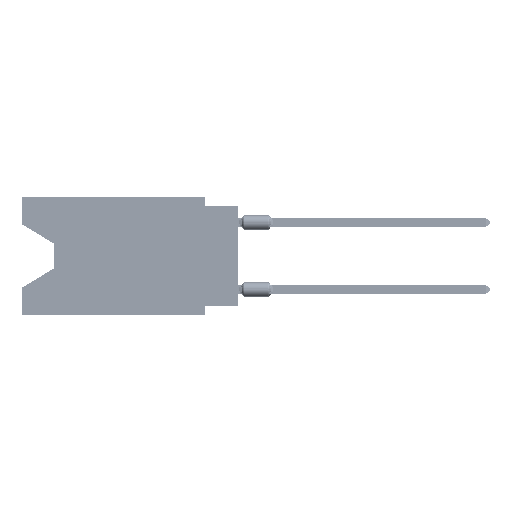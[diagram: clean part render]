
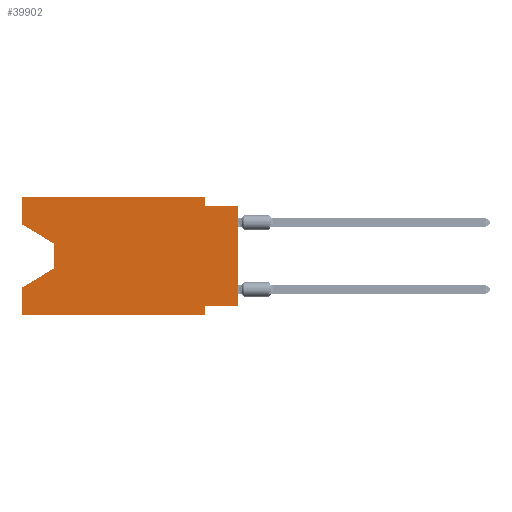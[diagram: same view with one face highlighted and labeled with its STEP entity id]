
A CAD part, left-side view. The second image highlights one B-rep face of the part: STEP entity #39902.
In plain terms, the highlighted planar face has unit normal (-1, 0, 0).
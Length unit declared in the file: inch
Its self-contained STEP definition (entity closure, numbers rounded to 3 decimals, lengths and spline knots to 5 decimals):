
#1618 = VERTEX_POINT ( 'NONE', #24203 ) ;
#2895 = VERTEX_POINT ( 'NONE', #55033 ) ;
#3774 = CARTESIAN_POINT ( 'NONE',  ( 0., 0.1, 0. ) ) ;
#4031 = EDGE_CURVE ( 'NONE', #2895, #60424, #76633, .T. ) ;
#6175 = CARTESIAN_POINT ( 'NONE',  ( 0., 0., -0.325 ) ) ;
#6309 = LINE ( 'NONE', #28253, #74478 ) ;
#8443 = CARTESIAN_POINT ( 'NONE',  ( 0., 0.645, 0. ) ) ;
#9538 = ORIENTED_EDGE ( 'NONE', *, *, #9828, .T. ) ;
#9793 = DIRECTION ( 'NONE',  ( 0., 0., -1. ) ) ;
#9828 = EDGE_CURVE ( 'NONE', #78543, #62343, #49968, .T. ) ;
#12840 = CARTESIAN_POINT ( 'NONE',  ( 0., 0.55, -0.212 ) ) ;
#13064 = CARTESIAN_POINT ( 'NONE',  ( 0., 0.645, -0.35 ) ) ;
#13562 = CARTESIAN_POINT ( 'NONE',  ( 0., 0.645, 0. ) ) ;
#14362 = EDGE_CURVE ( 'NONE', #1618, #95893, #100088, .T. ) ;
#14935 = CARTESIAN_POINT ( 'NONE',  ( 0., 0.645, -0.26975 ) ) ;
#19244 = CARTESIAN_POINT ( 'NONE',  ( 0., 0.1, -0.35 ) ) ;
#20510 = LINE ( 'NONE', #44009, #87578 ) ;
#20534 = DIRECTION ( 'NONE',  ( 0., 0., -1. ) ) ;
#21622 = EDGE_CURVE ( 'NONE', #34711, #39283, #20510, .T. ) ;
#21827 = DIRECTION ( 'NONE',  ( 0., -0.855, -0.519 ) ) ;
#22151 = ORIENTED_EDGE ( 'NONE', *, *, #102168, .T. ) ;
#22571 = DIRECTION ( 'NONE',  ( 0., 0., -1. ) ) ;
#22592 = DIRECTION ( 'NONE',  ( 1., 0., 0. ) ) ;
#23927 = CARTESIAN_POINT ( 'NONE',  ( 0., 0.55, -0.138 ) ) ;
#23942 = ORIENTED_EDGE ( 'NONE', *, *, #77847, .F. ) ;
#24137 = ORIENTED_EDGE ( 'NONE', *, *, #21622, .F. ) ;
#24203 = CARTESIAN_POINT ( 'NONE',  ( 0., 0.1, -0.025 ) ) ;
#26823 = ORIENTED_EDGE ( 'NONE', *, *, #64250, .F. ) ;
#28253 = CARTESIAN_POINT ( 'NONE',  ( 0., 0.1, 0. ) ) ;
#28830 = CARTESIAN_POINT ( 'NONE',  ( 0., 0., 0. ) ) ;
#29002 = DIRECTION ( 'NONE',  ( 0., -1., 0. ) ) ;
#29376 = CARTESIAN_POINT ( 'NONE',  ( 0., 0.55, -0.138 ) ) ;
#30294 = ORIENTED_EDGE ( 'NONE', *, *, #66082, .F. ) ;
#30373 = ORIENTED_EDGE ( 'NONE', *, *, #4031, .T. ) ;
#31202 = EDGE_CURVE ( 'NONE', #68637, #89518, #45872, .T. ) ;
#34433 = ORIENTED_EDGE ( 'NONE', *, *, #69255, .F. ) ;
#34711 = VERTEX_POINT ( 'NONE', #6175 ) ;
#35411 = VECTOR ( 'NONE', #78204, 39.37008 ) ;
#35824 = EDGE_CURVE ( 'NONE', #92430, #1618, #6309, .T. ) ;
#35868 = CARTESIAN_POINT ( 'NONE',  ( 0., 0., -0.025 ) ) ;
#36656 = DIRECTION ( 'NONE',  ( 0., 0., 1. ) ) ;
#39283 = VERTEX_POINT ( 'NONE', #44468 ) ;
#39902 = ADVANCED_FACE ( 'NONE', ( #101958 ), #77416, .F. ) ;
#40104 = LINE ( 'NONE', #23927, #66646 ) ;
#40309 = DIRECTION ( 'NONE',  ( 0., 0., 1. ) ) ;
#44009 = CARTESIAN_POINT ( 'NONE',  ( 0., 0., -0.325 ) ) ;
#44468 = CARTESIAN_POINT ( 'NONE',  ( 0., 0.1, -0.325 ) ) ;
#44953 = DIRECTION ( 'NONE',  ( 0., 0., -1. ) ) ;
#45872 = LINE ( 'NONE', #60480, #35411 ) ;
#48219 = ORIENTED_EDGE ( 'NONE', *, *, #35824, .F. ) ;
#49968 = LINE ( 'NONE', #96973, #67606 ) ;
#50547 = ORIENTED_EDGE ( 'NONE', *, *, #14362, .F. ) ;
#51049 = EDGE_LOOP ( 'NONE', ( #30373, #22151, #73092, #30294, #9538, #34433, #24137, #52480, #50547, #48219, #26823, #23942 ) ) ;
#51547 = CARTESIAN_POINT ( 'NONE',  ( 0., 0., -0.025 ) ) ;
#52480 = ORIENTED_EDGE ( 'NONE', *, *, #84926, .T. ) ;
#55033 = CARTESIAN_POINT ( 'NONE',  ( 0., 0.645, -0.08025 ) ) ;
#58853 = DIRECTION ( 'NONE',  ( 0., -1., 0. ) ) ;
#59265 = LINE ( 'NONE', #98446, #96436 ) ;
#60424 = VERTEX_POINT ( 'NONE', #29376 ) ;
#60480 = CARTESIAN_POINT ( 'NONE',  ( 0., 0.55, -0.212 ) ) ;
#62239 = LINE ( 'NONE', #94094, #80545 ) ;
#62343 = VERTEX_POINT ( 'NONE', #19244 ) ;
#62453 = CARTESIAN_POINT ( 'NONE',  ( 0., 0.645, 0. ) ) ;
#63295 = VECTOR ( 'NONE', #58853, 39.37008 ) ;
#64250 = EDGE_CURVE ( 'NONE', #83832, #92430, #59265, .T. ) ;
#66082 = EDGE_CURVE ( 'NONE', #78543, #89518, #79957, .T. ) ;
#66646 = VECTOR ( 'NONE', #9793, 39.37008 ) ;
#67606 = VECTOR ( 'NONE', #95434, 39.37008 ) ;
#68637 = VERTEX_POINT ( 'NONE', #12840 ) ;
#69015 = LINE ( 'NONE', #28830, #94339 ) ;
#69255 = EDGE_CURVE ( 'NONE', #39283, #62343, #62239, .T. ) ;
#73092 = ORIENTED_EDGE ( 'NONE', *, *, #31202, .T. ) ;
#73392 = VECTOR ( 'NONE', #40309, 39.37008 ) ;
#74478 = VECTOR ( 'NONE', #44953, 39.37008 ) ;
#75187 = VECTOR ( 'NONE', #77618, 39.37008 ) ;
#76633 = LINE ( 'NONE', #92312, #98126 ) ;
#77416 = PLANE ( 'NONE',  #98158 ) ;
#77618 = DIRECTION ( 'NONE',  ( 0., 0., 1. ) ) ;
#77847 = EDGE_CURVE ( 'NONE', #2895, #83832, #93809, .T. ) ;
#78204 = DIRECTION ( 'NONE',  ( 0., 0.855, -0.519 ) ) ;
#78543 = VERTEX_POINT ( 'NONE', #13064 ) ;
#79957 = LINE ( 'NONE', #8443, #73392 ) ;
#80545 = VECTOR ( 'NONE', #22571, 39.37008 ) ;
#83832 = VERTEX_POINT ( 'NONE', #13562 ) ;
#84211 = CARTESIAN_POINT ( 'NONE',  ( 0., 0.645, 0. ) ) ;
#84926 = EDGE_CURVE ( 'NONE', #34711, #95893, #69015, .T. ) ;
#87578 = VECTOR ( 'NONE', #98856, 39.37008 ) ;
#89518 = VERTEX_POINT ( 'NONE', #14935 ) ;
#92312 = CARTESIAN_POINT ( 'NONE',  ( 0., 0.645, -0.08025 ) ) ;
#92430 = VERTEX_POINT ( 'NONE', #3774 ) ;
#93809 = LINE ( 'NONE', #62453, #75187 ) ;
#94094 = CARTESIAN_POINT ( 'NONE',  ( 0., 0.1, -0.35 ) ) ;
#94339 = VECTOR ( 'NONE', #36656, 39.37008 ) ;
#95434 = DIRECTION ( 'NONE',  ( 0., -1., 0. ) ) ;
#95893 = VERTEX_POINT ( 'NONE', #35868 ) ;
#96436 = VECTOR ( 'NONE', #29002, 39.37008 ) ;
#96973 = CARTESIAN_POINT ( 'NONE',  ( 0., 0.645, -0.35 ) ) ;
#98126 = VECTOR ( 'NONE', #21827, 39.37008 ) ;
#98158 = AXIS2_PLACEMENT_3D ( 'NONE', #84211, #22592, #20534 ) ;
#98446 = CARTESIAN_POINT ( 'NONE',  ( 0., 0.645, 0. ) ) ;
#98856 = DIRECTION ( 'NONE',  ( 0., 1., 0. ) ) ;
#100088 = LINE ( 'NONE', #51547, #63295 ) ;
#101958 = FACE_OUTER_BOUND ( 'NONE', #51049, .T. ) ;
#102168 = EDGE_CURVE ( 'NONE', #60424, #68637, #40104, .T. ) ;
